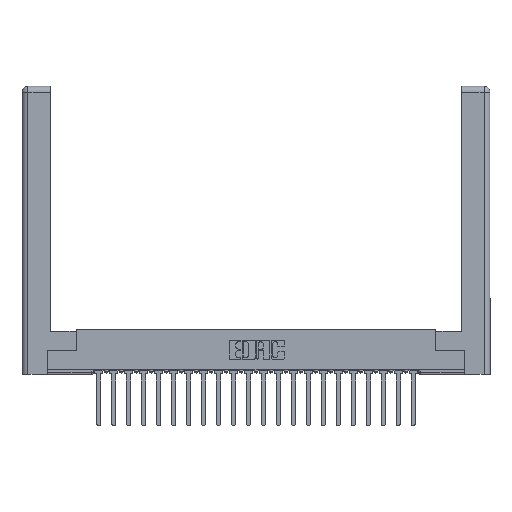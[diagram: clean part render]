
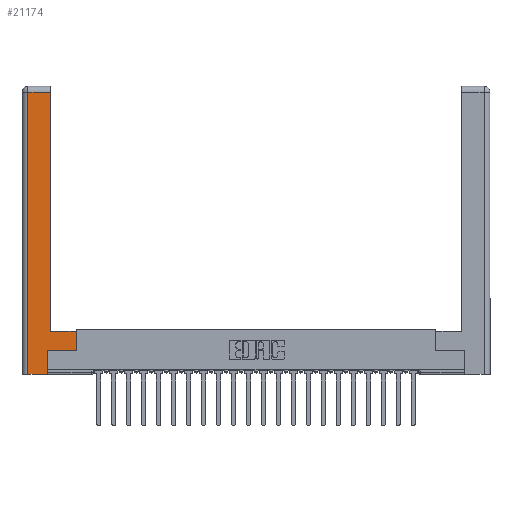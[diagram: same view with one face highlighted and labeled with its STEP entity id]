
A CAD part, top view. The second image highlights one B-rep face of the part: STEP entity #21174.
In plain terms, the highlighted planar face has unit normal (0, 0, 1).
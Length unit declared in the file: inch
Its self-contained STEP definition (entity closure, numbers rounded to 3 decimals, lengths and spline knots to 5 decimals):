
#145 = VERTEX_POINT ( 'NONE', #13265 ) ;
#189 = VECTOR ( 'NONE', #20747, 39.37008 ) ;
#328 = VERTEX_POINT ( 'NONE', #5118 ) ;
#483 = DIRECTION ( 'NONE',  ( 1., 0., 0. ) ) ;
#735 = CARTESIAN_POINT ( 'NONE',  ( 0.265, 0.245, 0. ) ) ;
#975 = VECTOR ( 'NONE', #18235, 39.37008 ) ;
#2431 = CARTESIAN_POINT ( 'NONE',  ( 0.295, 3., 0. ) ) ;
#2587 = DIRECTION ( 'NONE',  ( 0., 1., 0. ) ) ;
#2611 = ORIENTED_EDGE ( 'NONE', *, *, #5231, .T. ) ;
#2853 = LINE ( 'NONE', #21590, #22517 ) ;
#3125 = VERTEX_POINT ( 'NONE', #20520 ) ;
#3354 = CARTESIAN_POINT ( 'NONE',  ( 0.0615, 0., 0. ) ) ;
#3659 = CARTESIAN_POINT ( 'NONE',  ( 0.0615, 0., 0. ) ) ;
#3961 = LINE ( 'NONE', #3354, #22395 ) ;
#4111 = CARTESIAN_POINT ( 'NONE',  ( 0.565, 0.245, 0. ) ) ;
#4239 = DIRECTION ( 'NONE',  ( 0., 1., 0. ) ) ;
#4297 = PLANE ( 'NONE',  #19772 ) ;
#4347 = EDGE_CURVE ( 'NONE', #4687, #13552, #9253, .T. ) ;
#4687 = VERTEX_POINT ( 'NONE', #15954 ) ;
#5118 = CARTESIAN_POINT ( 'NONE',  ( 0.295, 2.94, 0. ) ) ;
#5231 = EDGE_CURVE ( 'NONE', #3125, #18601, #3961, .T. ) ;
#5278 = DIRECTION ( 'NONE',  ( 0., -1., 0. ) ) ;
#6936 = VECTOR ( 'NONE', #2587, 39.37008 ) ;
#7899 = CARTESIAN_POINT ( 'NONE',  ( 0.265, 0.245, 0. ) ) ;
#8160 = LINE ( 'NONE', #8655, #975 ) ;
#8655 = CARTESIAN_POINT ( 'NONE',  ( 0.0615, 2.94, 0. ) ) ;
#8656 = EDGE_CURVE ( 'NONE', #145, #12944, #2853, .T. ) ;
#8859 = EDGE_CURVE ( 'NONE', #12944, #20136, #11784, .T. ) ;
#9253 = LINE ( 'NONE', #7899, #17016 ) ;
#9624 = EDGE_CURVE ( 'NONE', #18601, #4687, #18030, .T. ) ;
#9837 = ORIENTED_EDGE ( 'NONE', *, *, #12521, .T. ) ;
#10661 = EDGE_CURVE ( 'NONE', #328, #3125, #8160, .T. ) ;
#10846 = CARTESIAN_POINT ( 'NONE',  ( 0.565, 0.45, 0. ) ) ;
#11747 = LINE ( 'NONE', #4111, #15969 ) ;
#11784 = LINE ( 'NONE', #24470, #189 ) ;
#11879 = ORIENTED_EDGE ( 'NONE', *, *, #4347, .T. ) ;
#12521 = EDGE_CURVE ( 'NONE', #20136, #328, #15570, .T. ) ;
#12944 = VERTEX_POINT ( 'NONE', #10846 ) ;
#13257 = ORIENTED_EDGE ( 'NONE', *, *, #9624, .T. ) ;
#13265 = CARTESIAN_POINT ( 'NONE',  ( 0.565, 0.245, 0. ) ) ;
#13465 = ORIENTED_EDGE ( 'NONE', *, *, #21837, .T. ) ;
#13552 = VERTEX_POINT ( 'NONE', #735 ) ;
#13564 = EDGE_LOOP ( 'NONE', ( #9837, #21580, #2611, #13257, #11879, #13465, #23798, #15421 ) ) ;
#13853 = DIRECTION ( 'NONE',  ( 0., 1., 0. ) ) ;
#15421 = ORIENTED_EDGE ( 'NONE', *, *, #8859, .T. ) ;
#15570 = LINE ( 'NONE', #2431, #6936 ) ;
#15954 = CARTESIAN_POINT ( 'NONE',  ( 0.265, 0., 0. ) ) ;
#15969 = VECTOR ( 'NONE', #483, 39.37008 ) ;
#16585 = CARTESIAN_POINT ( 'NONE',  ( 0.295, 0.45, 0. ) ) ;
#17016 = VECTOR ( 'NONE', #4239, 39.37008 ) ;
#18030 = LINE ( 'NONE', #22409, #19229 ) ;
#18235 = DIRECTION ( 'NONE',  ( -1., 0., 0. ) ) ;
#18601 = VERTEX_POINT ( 'NONE', #3659 ) ;
#18985 = FACE_OUTER_BOUND ( 'NONE', #13564, .T. ) ;
#19229 = VECTOR ( 'NONE', #22322, 39.37008 ) ;
#19438 = DIRECTION ( 'NONE',  ( -1., 0., 0. ) ) ;
#19772 = AXIS2_PLACEMENT_3D ( 'NONE', #21268, #23258, #19438 ) ;
#20136 = VERTEX_POINT ( 'NONE', #16585 ) ;
#20520 = CARTESIAN_POINT ( 'NONE',  ( 0.0615, 2.94, 0. ) ) ;
#20747 = DIRECTION ( 'NONE',  ( -1., 0., 0. ) ) ;
#21174 = ADVANCED_FACE ( 'NONE', ( #18985 ), #4297, .F. ) ;
#21268 = CARTESIAN_POINT ( 'NONE',  ( 0., 0., 0. ) ) ;
#21580 = ORIENTED_EDGE ( 'NONE', *, *, #10661, .T. ) ;
#21590 = CARTESIAN_POINT ( 'NONE',  ( 0.565, 0.45, 0. ) ) ;
#21837 = EDGE_CURVE ( 'NONE', #13552, #145, #11747, .T. ) ;
#22322 = DIRECTION ( 'NONE',  ( 1., 0., 0. ) ) ;
#22395 = VECTOR ( 'NONE', #5278, 39.37008 ) ;
#22409 = CARTESIAN_POINT ( 'NONE',  ( 0.265, 0., 0. ) ) ;
#22517 = VECTOR ( 'NONE', #13853, 39.37008 ) ;
#23258 = DIRECTION ( 'NONE',  ( 0., 0., -1. ) ) ;
#23798 = ORIENTED_EDGE ( 'NONE', *, *, #8656, .T. ) ;
#24470 = CARTESIAN_POINT ( 'NONE',  ( 0.295, 0.45, 0. ) ) ;
